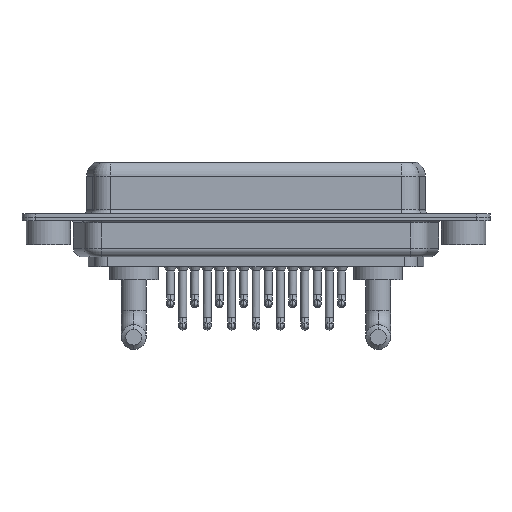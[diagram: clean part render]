
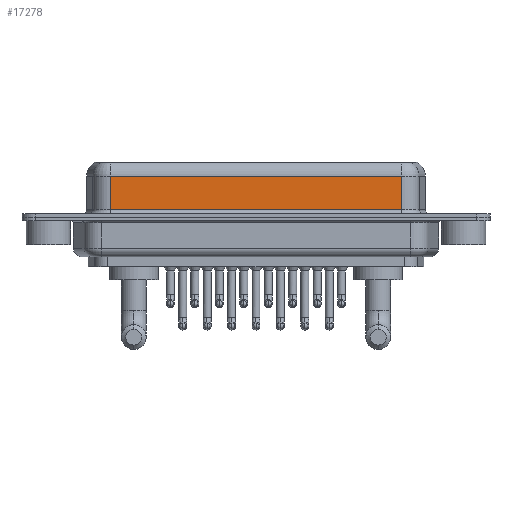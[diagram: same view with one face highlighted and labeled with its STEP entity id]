
A CAD part, front view. The second image highlights one B-rep face of the part: STEP entity #17278.
In plain terms, the highlighted planar face has unit normal (0, -1, 0).
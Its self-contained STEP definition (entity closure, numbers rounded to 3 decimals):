
#194 = EDGE_LOOP ( 'NONE', ( #1999, #16298, #2336, #19062 ) ) ;
#896 = VERTEX_POINT ( 'NONE', #3364 ) ;
#913 = CARTESIAN_POINT ( 'NONE',  ( 40.037, -3.95, 0.9 ) ) ;
#1999 = ORIENTED_EDGE ( 'NONE', *, *, #5999, .F. ) ;
#2235 = LINE ( 'NONE', #11946, #9196 ) ;
#2336 = ORIENTED_EDGE ( 'NONE', *, *, #8708, .T. ) ;
#2845 = DIRECTION ( 'NONE',  ( 0., 1., 0. ) ) ;
#2902 = EDGE_CURVE ( 'NONE', #16876, #13536, #16944, .T. ) ;
#3364 = CARTESIAN_POINT ( 'NONE',  ( 40.037, -3.95, 4.65 ) ) ;
#4733 = LINE ( 'NONE', #19085, #12356 ) ;
#5895 = VERTEX_POINT ( 'NONE', #19436 ) ;
#5931 = VECTOR ( 'NONE', #18933, 1000. ) ;
#5988 = VECTOR ( 'NONE', #13656, 1000. ) ;
#5999 = EDGE_CURVE ( 'NONE', #896, #13536, #2235, .T. ) ;
#7282 = DIRECTION ( 'NONE',  ( 0., 0., -1. ) ) ;
#8619 = CARTESIAN_POINT ( 'NONE',  ( 40.037, -3.95, 0.9 ) ) ;
#8708 = EDGE_CURVE ( 'NONE', #5895, #16876, #4733, .T. ) ;
#9196 = VECTOR ( 'NONE', #7282, 1000. ) ;
#9583 = CARTESIAN_POINT ( 'NONE',  ( 40.037, -3.95, 6.4 ) ) ;
#9686 = PLANE ( 'NONE',  #19068 ) ;
#11946 = CARTESIAN_POINT ( 'NONE',  ( 40.037, -3.95, 6.4 ) ) ;
#12356 = VECTOR ( 'NONE', #20658, 1000. ) ;
#12515 = CARTESIAN_POINT ( 'NONE',  ( 40.037, -3.95, 4.65 ) ) ;
#12561 = DIRECTION ( 'NONE',  ( 0., 0., 1. ) ) ;
#12665 = FACE_OUTER_BOUND ( 'NONE', #194, .T. ) ;
#13536 = VERTEX_POINT ( 'NONE', #8619 ) ;
#13656 = DIRECTION ( 'NONE',  ( 1., 0., 0. ) ) ;
#16298 = ORIENTED_EDGE ( 'NONE', *, *, #17687, .T. ) ;
#16868 = LINE ( 'NONE', #12515, #5931 ) ;
#16876 = VERTEX_POINT ( 'NONE', #19423 ) ;
#16944 = LINE ( 'NONE', #913, #5988 ) ;
#17278 = ADVANCED_FACE ( 'NONE', ( #12665 ), #9686, .F. ) ;
#17687 = EDGE_CURVE ( 'NONE', #896, #5895, #16868, .T. ) ;
#18933 = DIRECTION ( 'NONE',  ( -1., 0., 0. ) ) ;
#19062 = ORIENTED_EDGE ( 'NONE', *, *, #2902, .T. ) ;
#19068 = AXIS2_PLACEMENT_3D ( 'NONE', #9583, #2845, #12561 ) ;
#19085 = CARTESIAN_POINT ( 'NONE',  ( 7.013, -3.95, 6.4 ) ) ;
#19423 = CARTESIAN_POINT ( 'NONE',  ( 7.013, -3.95, 0.9 ) ) ;
#19436 = CARTESIAN_POINT ( 'NONE',  ( 7.013, -3.95, 4.65 ) ) ;
#20658 = DIRECTION ( 'NONE',  ( 0., 0., -1. ) ) ;
